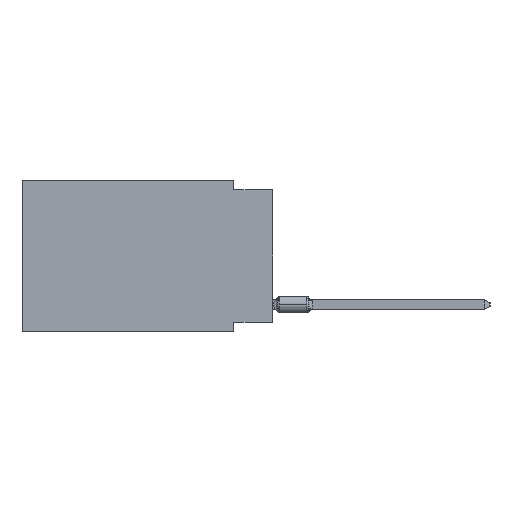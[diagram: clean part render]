
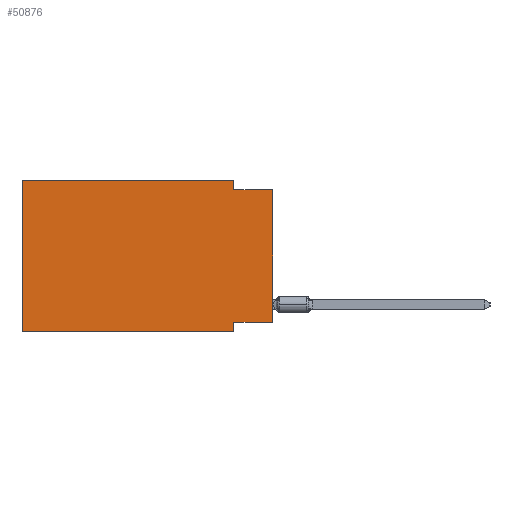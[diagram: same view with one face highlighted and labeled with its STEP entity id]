
A CAD part, left-side view. The second image highlights one B-rep face of the part: STEP entity #50876.
In plain terms, the highlighted planar face has unit normal (-1, 0, 0).
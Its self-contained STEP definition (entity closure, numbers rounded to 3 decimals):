
#1387 = VERTEX_POINT ( 'NONE', #52702 ) ;
#2891 = CARTESIAN_POINT ( 'NONE',  ( 0., 2.54, 0. ) ) ;
#4619 = DIRECTION ( 'NONE',  ( 0., 1., 0. ) ) ;
#4636 = EDGE_LOOP ( 'NONE', ( #36106, #46753, #68365, #24998, #47945, #43240, #64149, #24886 ) ) ;
#4861 = VECTOR ( 'NONE', #4619, 1000. ) ;
#6661 = LINE ( 'NONE', #12215, #47399 ) ;
#6947 = VECTOR ( 'NONE', #36889, 1000. ) ;
#7587 = VERTEX_POINT ( 'NONE', #25066 ) ;
#9249 = CARTESIAN_POINT ( 'NONE',  ( 0., 16.383, 0. ) ) ;
#9591 = DIRECTION ( 'NONE',  ( 0., 0., 1. ) ) ;
#10220 = VECTOR ( 'NONE', #39267, 1000. ) ;
#11306 = AXIS2_PLACEMENT_3D ( 'NONE', #68430, #37029, #58262 ) ;
#12215 = CARTESIAN_POINT ( 'NONE',  ( 0., 16.383, 0. ) ) ;
#13177 = LINE ( 'NONE', #35399, #39359 ) ;
#15771 = FACE_OUTER_BOUND ( 'NONE', #4636, .T. ) ;
#16779 = EDGE_CURVE ( 'NONE', #29988, #58190, #13177, .T. ) ;
#18585 = EDGE_CURVE ( 'NONE', #45544, #29988, #68743, .T. ) ;
#22367 = DIRECTION ( 'NONE',  ( 0., -1., 0. ) ) ;
#22909 = CARTESIAN_POINT ( 'NONE',  ( 0., 0., -0.635 ) ) ;
#24886 = ORIENTED_EDGE ( 'NONE', *, *, #18585, .F. ) ;
#24998 = ORIENTED_EDGE ( 'NONE', *, *, #25674, .F. ) ;
#25066 = CARTESIAN_POINT ( 'NONE',  ( 0., 0., -0.635 ) ) ;
#25674 = EDGE_CURVE ( 'NONE', #30713, #66718, #6661, .T. ) ;
#29988 = VERTEX_POINT ( 'NONE', #53542 ) ;
#30713 = VERTEX_POINT ( 'NONE', #39145 ) ;
#31811 = VERTEX_POINT ( 'NONE', #44902 ) ;
#33229 = LINE ( 'NONE', #53446, #51173 ) ;
#33385 = EDGE_CURVE ( 'NONE', #66718, #1387, #46687, .T. ) ;
#35399 = CARTESIAN_POINT ( 'NONE',  ( 0., 2.54, -9.906 ) ) ;
#36106 = ORIENTED_EDGE ( 'NONE', *, *, #58808, .T. ) ;
#36889 = DIRECTION ( 'NONE',  ( 0., 0., -1. ) ) ;
#37029 = DIRECTION ( 'NONE',  ( 1., 0., 0. ) ) ;
#39145 = CARTESIAN_POINT ( 'NONE',  ( 0., 16.383, 0. ) ) ;
#39267 = DIRECTION ( 'NONE',  ( 0., -1., 0. ) ) ;
#39359 = VECTOR ( 'NONE', #60571, 1000. ) ;
#39668 = CARTESIAN_POINT ( 'NONE',  ( 0., 0., -9.271 ) ) ;
#43240 = ORIENTED_EDGE ( 'NONE', *, *, #68503, .T. ) ;
#44902 = CARTESIAN_POINT ( 'NONE',  ( 0., 16.383, -9.906 ) ) ;
#45544 = VERTEX_POINT ( 'NONE', #39668 ) ;
#46687 = LINE ( 'NONE', #63717, #6947 ) ;
#46753 = ORIENTED_EDGE ( 'NONE', *, *, #50781, .F. ) ;
#47399 = VECTOR ( 'NONE', #22367, 1000. ) ;
#47945 = ORIENTED_EDGE ( 'NONE', *, *, #48085, .F. ) ;
#48085 = EDGE_CURVE ( 'NONE', #31811, #30713, #56642, .T. ) ;
#49254 = DIRECTION ( 'NONE',  ( 0., -1., 0. ) ) ;
#50121 = CARTESIAN_POINT ( 'NONE',  ( 0., 0., 0. ) ) ;
#50420 = CARTESIAN_POINT ( 'NONE',  ( 0., 0., -9.271 ) ) ;
#50781 = EDGE_CURVE ( 'NONE', #1387, #7587, #50782, .T. ) ;
#50782 = LINE ( 'NONE', #22909, #10220 ) ;
#50876 = ADVANCED_FACE ( 'NONE', ( #15771 ), #62844, .F. ) ;
#51173 = VECTOR ( 'NONE', #49254, 1000. ) ;
#52702 = CARTESIAN_POINT ( 'NONE',  ( 0., 2.54, -0.635 ) ) ;
#53446 = CARTESIAN_POINT ( 'NONE',  ( 0., 16.383, -9.906 ) ) ;
#53542 = CARTESIAN_POINT ( 'NONE',  ( 0., 2.54, -9.271 ) ) ;
#55341 = VECTOR ( 'NONE', #55666, 1000. ) ;
#55666 = DIRECTION ( 'NONE',  ( 0., 0., 1. ) ) ;
#56642 = LINE ( 'NONE', #9249, #58784 ) ;
#58190 = VERTEX_POINT ( 'NONE', #63533 ) ;
#58262 = DIRECTION ( 'NONE',  ( 0., 0., -1. ) ) ;
#58784 = VECTOR ( 'NONE', #9591, 1000. ) ;
#58808 = EDGE_CURVE ( 'NONE', #45544, #7587, #67166, .T. ) ;
#60571 = DIRECTION ( 'NONE',  ( 0., 0., -1. ) ) ;
#62844 = PLANE ( 'NONE',  #11306 ) ;
#63533 = CARTESIAN_POINT ( 'NONE',  ( 0., 2.54, -9.906 ) ) ;
#63717 = CARTESIAN_POINT ( 'NONE',  ( 0., 2.54, 0. ) ) ;
#64149 = ORIENTED_EDGE ( 'NONE', *, *, #16779, .F. ) ;
#66718 = VERTEX_POINT ( 'NONE', #2891 ) ;
#67166 = LINE ( 'NONE', #50121, #55341 ) ;
#68365 = ORIENTED_EDGE ( 'NONE', *, *, #33385, .F. ) ;
#68430 = CARTESIAN_POINT ( 'NONE',  ( 0., 16.383, 0. ) ) ;
#68503 = EDGE_CURVE ( 'NONE', #31811, #58190, #33229, .T. ) ;
#68743 = LINE ( 'NONE', #50420, #4861 ) ;
